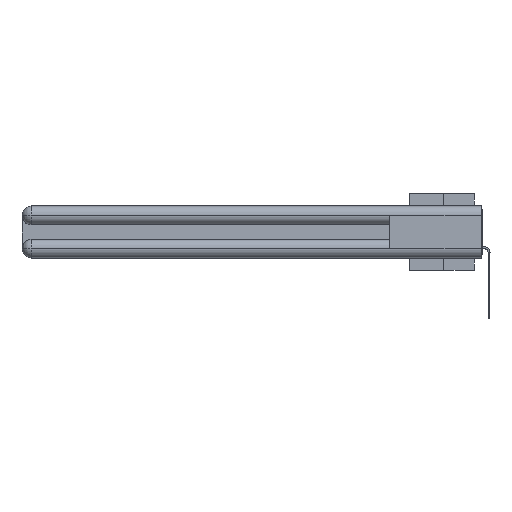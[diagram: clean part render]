
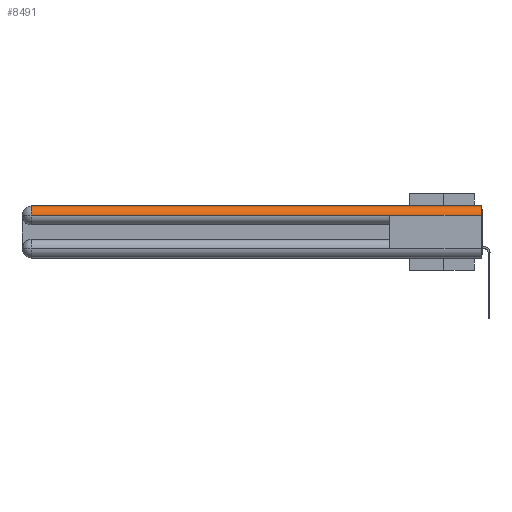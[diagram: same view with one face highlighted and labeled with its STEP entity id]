
A CAD part, left-side view. The second image highlights one B-rep face of the part: STEP entity #8491.
In plain terms, the highlighted cylindrical face has radius 1.562 mm (diameter 3.124 mm), a partial arc.
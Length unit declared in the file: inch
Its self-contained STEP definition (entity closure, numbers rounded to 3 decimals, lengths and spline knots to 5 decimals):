
#158 = CIRCLE ( 'NONE', #4430, 0.0615 ) ;
#1508 = ORIENTED_EDGE ( 'NONE', *, *, #4017, .F. ) ;
#2838 = AXIS2_PLACEMENT_3D ( 'NONE', #25368, #12744, #23047 ) ;
#2975 = VERTEX_POINT ( 'NONE', #18981 ) ;
#3327 = DIRECTION ( 'NONE',  ( 1., 0., 0. ) ) ;
#3656 = CARTESIAN_POINT ( 'NONE',  ( 0.0615, 0., -0.0615 ) ) ;
#4017 = EDGE_CURVE ( 'NONE', #31132, #2975, #19564, .T. ) ;
#4283 = DIRECTION ( 'NONE',  ( 0., -1., 0. ) ) ;
#4430 = AXIS2_PLACEMENT_3D ( 'NONE', #19266, #4283, #14437 ) ;
#5114 = VERTEX_POINT ( 'NONE', #26198 ) ;
#5180 = DIRECTION ( 'NONE',  ( 0., -1., 0. ) ) ;
#7873 = CARTESIAN_POINT ( 'NONE',  ( 0.0615, 0., 0. ) ) ;
#8491 = ADVANCED_FACE ( 'NONE', ( #30352 ), #10423, .T. ) ;
#8588 = LINE ( 'NONE', #25564, #11308 ) ;
#8937 = EDGE_CURVE ( 'NONE', #5114, #31132, #20614, .T. ) ;
#9635 = EDGE_CURVE ( 'NONE', #25399, #21821, #158, .T. ) ;
#10423 = CYLINDRICAL_SURFACE ( 'NONE', #2838, 0.0615 ) ;
#11308 = VECTOR ( 'NONE', #28052, 39.37008 ) ;
#11338 = EDGE_LOOP ( 'NONE', ( #19274, #31881, #19429, #1508, #24051 ) ) ;
#12402 = CARTESIAN_POINT ( 'NONE',  ( 0., 3., -0.0615 ) ) ;
#12744 = DIRECTION ( 'NONE',  ( 0., 1., 0. ) ) ;
#12997 = CARTESIAN_POINT ( 'NONE',  ( 0.0615, 2.94, 0. ) ) ;
#13310 = CARTESIAN_POINT ( 'NONE',  ( 0., 0., -0.0615 ) ) ;
#14437 = DIRECTION ( 'NONE',  ( 0., 0., 1. ) ) ;
#16891 = AXIS2_PLACEMENT_3D ( 'NONE', #3656, #31262, #3327 ) ;
#17035 = CARTESIAN_POINT ( 'NONE',  ( 0., 2.94, -0.0615 ) ) ;
#18726 = VECTOR ( 'NONE', #5180, 39.37008 ) ;
#18981 = CARTESIAN_POINT ( 'NONE',  ( 0., 0.6, -0.0615 ) ) ;
#19266 = CARTESIAN_POINT ( 'NONE',  ( 0.0615, 2.94, -0.0615 ) ) ;
#19274 = ORIENTED_EDGE ( 'NONE', *, *, #20741, .F. ) ;
#19429 = ORIENTED_EDGE ( 'NONE', *, *, #29710, .T. ) ;
#19564 = LINE ( 'NONE', #12402, #20878 ) ;
#19990 = LINE ( 'NONE', #7873, #18726 ) ;
#20209 = DIRECTION ( 'NONE',  ( 0., 1., 0. ) ) ;
#20614 = CIRCLE ( 'NONE', #16891, 0.0615 ) ;
#20741 = EDGE_CURVE ( 'NONE', #25399, #5114, #19990, .T. ) ;
#20878 = VECTOR ( 'NONE', #20209, 39.37008 ) ;
#21821 = VERTEX_POINT ( 'NONE', #17035 ) ;
#23047 = DIRECTION ( 'NONE',  ( 0., 0., 1. ) ) ;
#24051 = ORIENTED_EDGE ( 'NONE', *, *, #8937, .F. ) ;
#25368 = CARTESIAN_POINT ( 'NONE',  ( 0.0615, 0., -0.0615 ) ) ;
#25399 = VERTEX_POINT ( 'NONE', #12997 ) ;
#25564 = CARTESIAN_POINT ( 'NONE',  ( 0., 3., -0.0615 ) ) ;
#26198 = CARTESIAN_POINT ( 'NONE',  ( 0.0615, 0., 0. ) ) ;
#28052 = DIRECTION ( 'NONE',  ( 0., -1., 0. ) ) ;
#29710 = EDGE_CURVE ( 'NONE', #21821, #2975, #8588, .T. ) ;
#30352 = FACE_OUTER_BOUND ( 'NONE', #11338, .T. ) ;
#31132 = VERTEX_POINT ( 'NONE', #13310 ) ;
#31262 = DIRECTION ( 'NONE',  ( 0., -1., 0. ) ) ;
#31881 = ORIENTED_EDGE ( 'NONE', *, *, #9635, .T. ) ;
